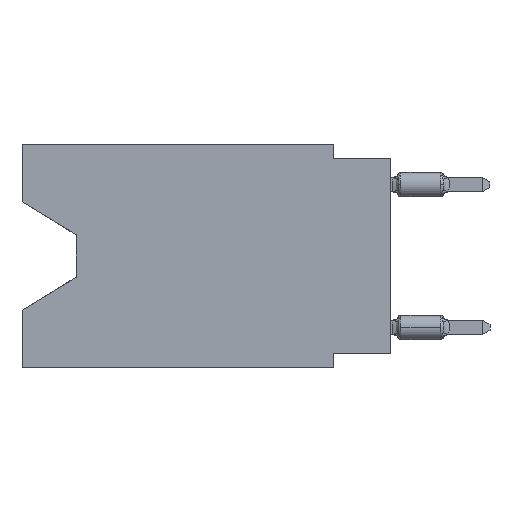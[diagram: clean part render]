
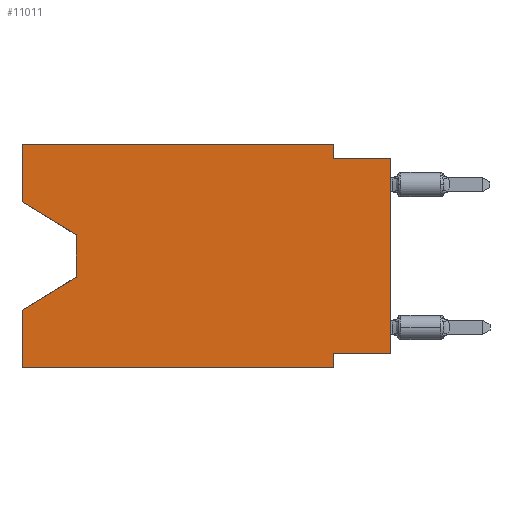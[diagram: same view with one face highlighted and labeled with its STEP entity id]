
A CAD part, left-side view. The second image highlights one B-rep face of the part: STEP entity #11011.
In plain terms, the highlighted planar face has unit normal (-1, 0, 0).
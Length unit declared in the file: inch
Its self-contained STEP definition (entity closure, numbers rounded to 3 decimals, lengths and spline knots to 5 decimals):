
#390 = DIRECTION ( 'NONE',  ( 0., 0., 1. ) ) ;
#478 = CARTESIAN_POINT ( 'NONE',  ( 0., 0.645, 0. ) ) ;
#1538 = DIRECTION ( 'NONE',  ( 0., -1., 0. ) ) ;
#1554 = DIRECTION ( 'NONE',  ( 0., 0., -1. ) ) ;
#3162 = EDGE_CURVE ( 'NONE', #48788, #23227, #26495, .T. ) ;
#4031 = VECTOR ( 'NONE', #1538, 39.37008 ) ;
#4652 = VERTEX_POINT ( 'NONE', #46966 ) ;
#4949 = ORIENTED_EDGE ( 'NONE', *, *, #13887, .F. ) ;
#5764 = CARTESIAN_POINT ( 'NONE',  ( 0., 0.1, -0.39 ) ) ;
#6538 = VERTEX_POINT ( 'NONE', #29003 ) ;
#6939 = EDGE_CURVE ( 'NONE', #52110, #29267, #37314, .T. ) ;
#8073 = DIRECTION ( 'NONE',  ( 0., -1., 0. ) ) ;
#11011 = ADVANCED_FACE ( 'NONE', ( #30488 ), #27325, .F. ) ;
#11490 = EDGE_CURVE ( 'NONE', #20282, #12641, #15781, .T. ) ;
#11548 = EDGE_CURVE ( 'NONE', #6538, #25864, #45968, .T. ) ;
#11865 = AXIS2_PLACEMENT_3D ( 'NONE', #14465, #40473, #23122 ) ;
#12641 = VERTEX_POINT ( 'NONE', #41554 ) ;
#13887 = EDGE_CURVE ( 'NONE', #52110, #50295, #30048, .T. ) ;
#13999 = CARTESIAN_POINT ( 'NONE',  ( 0., 0.1, -0.025 ) ) ;
#14349 = CARTESIAN_POINT ( 'NONE',  ( 0., 0., 0. ) ) ;
#14465 = CARTESIAN_POINT ( 'NONE',  ( 0., 0.645, 0. ) ) ;
#14534 = VECTOR ( 'NONE', #8073, 39.37008 ) ;
#15529 = DIRECTION ( 'NONE',  ( 0., -0.855, -0.519 ) ) ;
#15781 = LINE ( 'NONE', #37574, #16752 ) ;
#16009 = ORIENTED_EDGE ( 'NONE', *, *, #30334, .F. ) ;
#16752 = VECTOR ( 'NONE', #19983, 39.37008 ) ;
#16953 = VECTOR ( 'NONE', #390, 39.37008 ) ;
#19983 = DIRECTION ( 'NONE',  ( 0., 1., 0. ) ) ;
#20134 = LINE ( 'NONE', #20944, #14534 ) ;
#20146 = EDGE_CURVE ( 'NONE', #29267, #20271, #20866, .T. ) ;
#20271 = VERTEX_POINT ( 'NONE', #43248 ) ;
#20282 = VERTEX_POINT ( 'NONE', #30107 ) ;
#20793 = VECTOR ( 'NONE', #15529, 39.37008 ) ;
#20866 = LINE ( 'NONE', #31462, #42984 ) ;
#20944 = CARTESIAN_POINT ( 'NONE',  ( 0., 0.645, 0. ) ) ;
#21653 = CARTESIAN_POINT ( 'NONE',  ( 0., 0., -0.025 ) ) ;
#21939 = CARTESIAN_POINT ( 'NONE',  ( 0., 0.645, 0. ) ) ;
#22170 = ORIENTED_EDGE ( 'NONE', *, *, #20146, .T. ) ;
#23122 = DIRECTION ( 'NONE',  ( 0., 0., -1. ) ) ;
#23227 = VERTEX_POINT ( 'NONE', #26427 ) ;
#24720 = DIRECTION ( 'NONE',  ( 0., 0., -1. ) ) ;
#25864 = VERTEX_POINT ( 'NONE', #13999 ) ;
#25933 = CARTESIAN_POINT ( 'NONE',  ( 0., 0.645, -0.39 ) ) ;
#26374 = EDGE_CURVE ( 'NONE', #12641, #23227, #35111, .T. ) ;
#26427 = CARTESIAN_POINT ( 'NONE',  ( 0., 0.1, -0.39 ) ) ;
#26495 = LINE ( 'NONE', #25933, #51969 ) ;
#26581 = VECTOR ( 'NONE', #24720, 39.37008 ) ;
#27325 = PLANE ( 'NONE',  #11865 ) ;
#27329 = ORIENTED_EDGE ( 'NONE', *, *, #33252, .F. ) ;
#27509 = EDGE_CURVE ( 'NONE', #50295, #6538, #20134, .T. ) ;
#28534 = VERTEX_POINT ( 'NONE', #29038 ) ;
#28938 = CARTESIAN_POINT ( 'NONE',  ( 0., 0.645, -0.10025 ) ) ;
#29003 = CARTESIAN_POINT ( 'NONE',  ( 0., 0.1, 0. ) ) ;
#29038 = CARTESIAN_POINT ( 'NONE',  ( 0., 0., -0.025 ) ) ;
#29108 = CARTESIAN_POINT ( 'NONE',  ( 0., 0.55, -0.158 ) ) ;
#29267 = VERTEX_POINT ( 'NONE', #29108 ) ;
#30048 = LINE ( 'NONE', #21939, #38268 ) ;
#30107 = CARTESIAN_POINT ( 'NONE',  ( 0., 0., -0.365 ) ) ;
#30259 = ORIENTED_EDGE ( 'NONE', *, *, #45492, .T. ) ;
#30334 = EDGE_CURVE ( 'NONE', #25864, #28534, #44020, .T. ) ;
#30420 = DIRECTION ( 'NONE',  ( 0., -1., 0. ) ) ;
#30488 = FACE_OUTER_BOUND ( 'NONE', #39860, .T. ) ;
#31222 = ORIENTED_EDGE ( 'NONE', *, *, #6939, .T. ) ;
#31462 = CARTESIAN_POINT ( 'NONE',  ( 0., 0.55, -0.158 ) ) ;
#33014 = CARTESIAN_POINT ( 'NONE',  ( 0., 0.645, -0.39 ) ) ;
#33252 = EDGE_CURVE ( 'NONE', #48788, #4652, #50791, .T. ) ;
#34982 = ORIENTED_EDGE ( 'NONE', *, *, #11548, .F. ) ;
#35111 = LINE ( 'NONE', #5764, #40851 ) ;
#37314 = LINE ( 'NONE', #28938, #20793 ) ;
#37574 = CARTESIAN_POINT ( 'NONE',  ( 0., 0., -0.365 ) ) ;
#38268 = VECTOR ( 'NONE', #38438, 39.37008 ) ;
#38403 = LINE ( 'NONE', #38694, #53632 ) ;
#38438 = DIRECTION ( 'NONE',  ( 0., 0., 1. ) ) ;
#38694 = CARTESIAN_POINT ( 'NONE',  ( 0., 0.55, -0.232 ) ) ;
#39055 = DIRECTION ( 'NONE',  ( 0., 0., 1. ) ) ;
#39171 = ORIENTED_EDGE ( 'NONE', *, *, #3162, .T. ) ;
#39860 = EDGE_LOOP ( 'NONE', ( #31222, #22170, #30259, #27329, #39171, #45497, #44717, #46895, #16009, #34982, #53313, #4949 ) ) ;
#40473 = DIRECTION ( 'NONE',  ( 1., 0., 0. ) ) ;
#40851 = VECTOR ( 'NONE', #1554, 39.37008 ) ;
#41554 = CARTESIAN_POINT ( 'NONE',  ( 0., 0.1, -0.365 ) ) ;
#42984 = VECTOR ( 'NONE', #48520, 39.37008 ) ;
#43248 = CARTESIAN_POINT ( 'NONE',  ( 0., 0.55, -0.232 ) ) ;
#44020 = LINE ( 'NONE', #21653, #4031 ) ;
#44411 = EDGE_CURVE ( 'NONE', #20282, #28534, #51801, .T. ) ;
#44717 = ORIENTED_EDGE ( 'NONE', *, *, #11490, .F. ) ;
#45492 = EDGE_CURVE ( 'NONE', #20271, #4652, #38403, .T. ) ;
#45497 = ORIENTED_EDGE ( 'NONE', *, *, #26374, .F. ) ;
#45968 = LINE ( 'NONE', #54604, #26581 ) ;
#46895 = ORIENTED_EDGE ( 'NONE', *, *, #44411, .T. ) ;
#46966 = CARTESIAN_POINT ( 'NONE',  ( 0., 0.645, -0.28975 ) ) ;
#47064 = DIRECTION ( 'NONE',  ( 0., 0.855, -0.519 ) ) ;
#47589 = CARTESIAN_POINT ( 'NONE',  ( 0., 0.645, 0. ) ) ;
#47882 = VECTOR ( 'NONE', #39055, 39.37008 ) ;
#48520 = DIRECTION ( 'NONE',  ( 0., 0., -1. ) ) ;
#48788 = VERTEX_POINT ( 'NONE', #33014 ) ;
#50295 = VERTEX_POINT ( 'NONE', #47589 ) ;
#50791 = LINE ( 'NONE', #478, #47882 ) ;
#51792 = CARTESIAN_POINT ( 'NONE',  ( 0., 0.645, -0.10025 ) ) ;
#51801 = LINE ( 'NONE', #14349, #16953 ) ;
#51969 = VECTOR ( 'NONE', #30420, 39.37008 ) ;
#52110 = VERTEX_POINT ( 'NONE', #51792 ) ;
#53313 = ORIENTED_EDGE ( 'NONE', *, *, #27509, .F. ) ;
#53632 = VECTOR ( 'NONE', #47064, 39.37008 ) ;
#54604 = CARTESIAN_POINT ( 'NONE',  ( 0., 0.1, 0. ) ) ;
